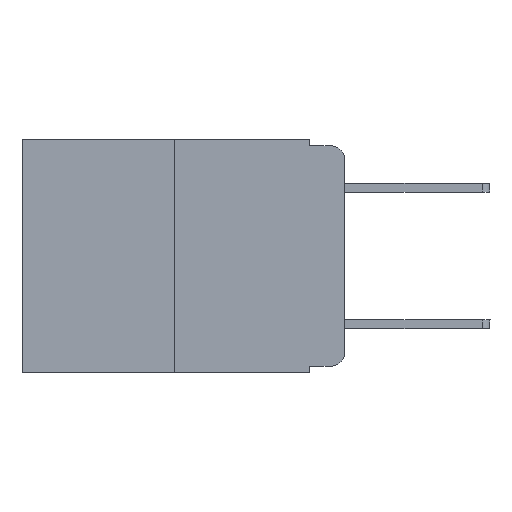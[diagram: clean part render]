
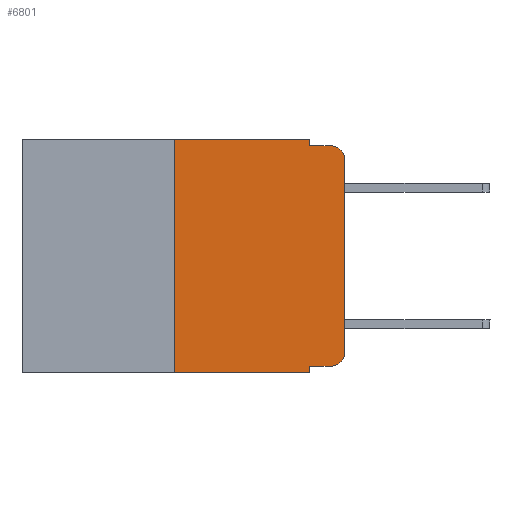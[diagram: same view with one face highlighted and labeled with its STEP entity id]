
A CAD part, left-side view. The second image highlights one B-rep face of the part: STEP entity #6801.
In plain terms, the highlighted planar face has unit normal (-1, 0, 0).
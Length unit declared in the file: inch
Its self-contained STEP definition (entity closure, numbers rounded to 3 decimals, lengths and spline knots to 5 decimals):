
#11 = ORIENTED_EDGE ( 'NONE', *, *, #679, .F. ) ;
#95 = LINE ( 'NONE', #8951, #6749 ) ;
#194 = EDGE_CURVE ( 'NONE', #4984, #8080, #4627, .T. ) ;
#457 = ORIENTED_EDGE ( 'NONE', *, *, #13848, .T. ) ;
#589 = ORIENTED_EDGE ( 'NONE', *, *, #4780, .T. ) ;
#653 = DIRECTION ( 'NONE',  ( 0., 0., 1. ) ) ;
#679 = EDGE_CURVE ( 'NONE', #11073, #1360, #14571, .T. ) ;
#1066 = CARTESIAN_POINT ( 'NONE',  ( 0., 0.051, 0. ) ) ;
#1102 = DIRECTION ( 'NONE',  ( -1., 0., 0. ) ) ;
#1360 = VERTEX_POINT ( 'NONE', #12757 ) ;
#1574 = ORIENTED_EDGE ( 'NONE', *, *, #5342, .F. ) ;
#1752 = CARTESIAN_POINT ( 'NONE',  ( 0., 0.051, -0.343 ) ) ;
#1989 = DIRECTION ( 'NONE',  ( -1., 0., 0. ) ) ;
#2016 = DIRECTION ( 'NONE',  ( 0., 0., -1. ) ) ;
#2070 = DIRECTION ( 'NONE',  ( 0., 0., -1. ) ) ;
#2204 = CARTESIAN_POINT ( 'NONE',  ( 0., 0.25, -0.343 ) ) ;
#2240 = VECTOR ( 'NONE', #9226, 39.37008 ) ;
#2386 = CIRCLE ( 'NONE', #2653, 0.02 ) ;
#2431 = EDGE_LOOP ( 'NONE', ( #7576, #457, #6761, #11, #11940, #5987, #7184, #1574, #589, #4022 ) ) ;
#2653 = AXIS2_PLACEMENT_3D ( 'NONE', #11165, #1102, #5984 ) ;
#2950 = VECTOR ( 'NONE', #11380, 39.37008 ) ;
#3179 = CARTESIAN_POINT ( 'NONE',  ( 0., 0., -0.03 ) ) ;
#3340 = CARTESIAN_POINT ( 'NONE',  ( 0., 0.051, -0.01 ) ) ;
#3877 = CARTESIAN_POINT ( 'NONE',  ( 0., 0.02, -0.01 ) ) ;
#4022 = ORIENTED_EDGE ( 'NONE', *, *, #6318, .T. ) ;
#4082 = VERTEX_POINT ( 'NONE', #1752 ) ;
#4627 = LINE ( 'NONE', #13347, #14587 ) ;
#4780 = EDGE_CURVE ( 'NONE', #8997, #12627, #12148, .T. ) ;
#4984 = VERTEX_POINT ( 'NONE', #2204 ) ;
#5342 = EDGE_CURVE ( 'NONE', #8997, #4082, #5432, .T. ) ;
#5432 = LINE ( 'NONE', #8970, #2240 ) ;
#5711 = EDGE_CURVE ( 'NONE', #4984, #4082, #95, .T. ) ;
#5797 = VECTOR ( 'NONE', #11241, 39.37008 ) ;
#5893 = DIRECTION ( 'NONE',  ( 0., -1., 0. ) ) ;
#5984 = DIRECTION ( 'NONE',  ( 0., 0., -1. ) ) ;
#5987 = ORIENTED_EDGE ( 'NONE', *, *, #194, .F. ) ;
#6194 = VECTOR ( 'NONE', #5893, 39.37008 ) ;
#6318 = EDGE_CURVE ( 'NONE', #12627, #13225, #10172, .T. ) ;
#6563 = DIRECTION ( 'NONE',  ( 0., -1., 0. ) ) ;
#6623 = CARTESIAN_POINT ( 'NONE',  ( 0., 0.02, -0.333 ) ) ;
#6749 = VECTOR ( 'NONE', #6563, 39.37008 ) ;
#6761 = ORIENTED_EDGE ( 'NONE', *, *, #15533, .F. ) ;
#6801 = ADVANCED_FACE ( 'NONE', ( #12114 ), #12416, .F. ) ;
#6881 = CARTESIAN_POINT ( 'NONE',  ( 0., 0.02, -0.313 ) ) ;
#7104 = CARTESIAN_POINT ( 'NONE',  ( 0., 0.473, 0. ) ) ;
#7160 = VECTOR ( 'NONE', #15936, 39.37008 ) ;
#7184 = ORIENTED_EDGE ( 'NONE', *, *, #5711, .T. ) ;
#7209 = LINE ( 'NONE', #3340, #7160 ) ;
#7576 = ORIENTED_EDGE ( 'NONE', *, *, #12079, .T. ) ;
#7609 = LINE ( 'NONE', #12607, #2950 ) ;
#7796 = LINE ( 'NONE', #13800, #5797 ) ;
#7846 = VERTEX_POINT ( 'NONE', #3877 ) ;
#8080 = VERTEX_POINT ( 'NONE', #15591 ) ;
#8495 = DIRECTION ( 'NONE',  ( 1., 0., 0. ) ) ;
#8951 = CARTESIAN_POINT ( 'NONE',  ( 0., 0.473, -0.343 ) ) ;
#8970 = CARTESIAN_POINT ( 'NONE',  ( 0., 0.051, 0. ) ) ;
#8997 = VERTEX_POINT ( 'NONE', #13714 ) ;
#9226 = DIRECTION ( 'NONE',  ( 0., 0., -1. ) ) ;
#10172 = CIRCLE ( 'NONE', #13067, 0.02 ) ;
#10891 = VECTOR ( 'NONE', #2016, 39.37008 ) ;
#10901 = CARTESIAN_POINT ( 'NONE',  ( 0., 0.051, -0.333 ) ) ;
#11073 = VERTEX_POINT ( 'NONE', #1066 ) ;
#11165 = CARTESIAN_POINT ( 'NONE',  ( 0., 0.02, -0.03 ) ) ;
#11241 = DIRECTION ( 'NONE',  ( 0., 0., 1. ) ) ;
#11380 = DIRECTION ( 'NONE',  ( 0., -1., 0. ) ) ;
#11940 = ORIENTED_EDGE ( 'NONE', *, *, #15751, .F. ) ;
#12079 = EDGE_CURVE ( 'NONE', #13225, #15426, #7796, .T. ) ;
#12114 = FACE_OUTER_BOUND ( 'NONE', #2431, .T. ) ;
#12148 = LINE ( 'NONE', #10901, #6194 ) ;
#12416 = PLANE ( 'NONE',  #12548 ) ;
#12548 = AXIS2_PLACEMENT_3D ( 'NONE', #7104, #8495, #13581 ) ;
#12607 = CARTESIAN_POINT ( 'NONE',  ( 0., 0.473, 0. ) ) ;
#12627 = VERTEX_POINT ( 'NONE', #6623 ) ;
#12757 = CARTESIAN_POINT ( 'NONE',  ( 0., 0.051, -0.01 ) ) ;
#13067 = AXIS2_PLACEMENT_3D ( 'NONE', #6881, #1989, #2070 ) ;
#13225 = VERTEX_POINT ( 'NONE', #13336 ) ;
#13336 = CARTESIAN_POINT ( 'NONE',  ( 0., 0., -0.313 ) ) ;
#13347 = CARTESIAN_POINT ( 'NONE',  ( 0., 0.25, 0. ) ) ;
#13581 = DIRECTION ( 'NONE',  ( 0., 0., -1. ) ) ;
#13714 = CARTESIAN_POINT ( 'NONE',  ( 0., 0.051, -0.333 ) ) ;
#13800 = CARTESIAN_POINT ( 'NONE',  ( 0., 0., 0. ) ) ;
#13848 = EDGE_CURVE ( 'NONE', #15426, #7846, #2386, .T. ) ;
#14571 = LINE ( 'NONE', #14791, #10891 ) ;
#14587 = VECTOR ( 'NONE', #653, 39.37008 ) ;
#14791 = CARTESIAN_POINT ( 'NONE',  ( 0., 0.051, 0. ) ) ;
#15426 = VERTEX_POINT ( 'NONE', #3179 ) ;
#15533 = EDGE_CURVE ( 'NONE', #1360, #7846, #7209, .T. ) ;
#15591 = CARTESIAN_POINT ( 'NONE',  ( 0., 0.25, 0. ) ) ;
#15751 = EDGE_CURVE ( 'NONE', #8080, #11073, #7609, .T. ) ;
#15936 = DIRECTION ( 'NONE',  ( 0., -1., 0. ) ) ;
